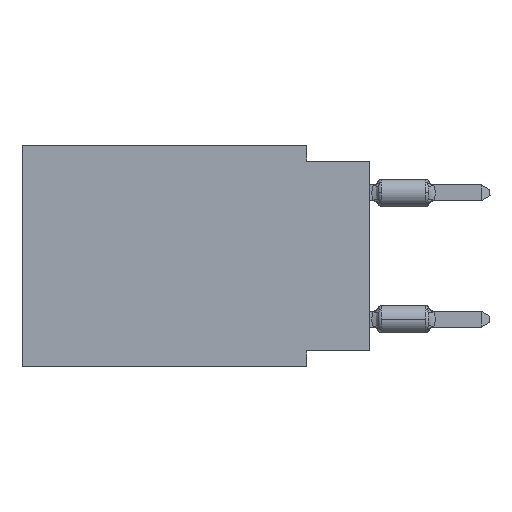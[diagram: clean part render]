
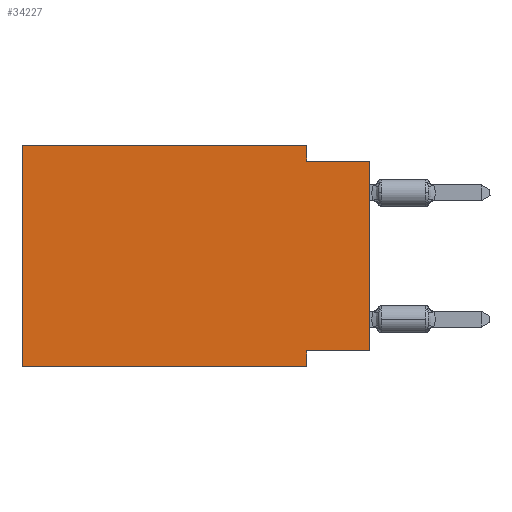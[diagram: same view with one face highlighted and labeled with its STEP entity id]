
A CAD part, left-side view. The second image highlights one B-rep face of the part: STEP entity #34227.
In plain terms, the highlighted planar face has unit normal (-1, 0, 0).
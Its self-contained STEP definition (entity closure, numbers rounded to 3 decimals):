
#984 = EDGE_CURVE ( 'NONE', #47885, #24901, #5481, .T. ) ;
#1467 = LINE ( 'NONE', #22035, #21610 ) ;
#1896 = PLANE ( 'NONE',  #51335 ) ;
#1960 = VERTEX_POINT ( 'NONE', #10460 ) ;
#2420 = FACE_OUTER_BOUND ( 'NONE', #35172, .T. ) ;
#2881 = VECTOR ( 'NONE', #37565, 1000. ) ;
#5127 = CARTESIAN_POINT ( 'NONE',  ( 0., 0., 0. ) ) ;
#5481 = LINE ( 'NONE', #21591, #23603 ) ;
#6305 = EDGE_CURVE ( 'NONE', #47885, #1960, #35040, .T. ) ;
#7955 = CARTESIAN_POINT ( 'NONE',  ( 0., 0., -0.635 ) ) ;
#8217 = CARTESIAN_POINT ( 'NONE',  ( 0., 0., -0.635 ) ) ;
#8836 = CARTESIAN_POINT ( 'NONE',  ( 0., 13.97, 0. ) ) ;
#9894 = DIRECTION ( 'NONE',  ( 0., 0., -1. ) ) ;
#10460 = CARTESIAN_POINT ( 'NONE',  ( 0., 2.54, -8.89 ) ) ;
#12663 = DIRECTION ( 'NONE',  ( 0., -1., 0. ) ) ;
#13240 = VERTEX_POINT ( 'NONE', #26535 ) ;
#14317 = EDGE_CURVE ( 'NONE', #24901, #13240, #45087, .T. ) ;
#15004 = DIRECTION ( 'NONE',  ( 0., -1., 0. ) ) ;
#16080 = CARTESIAN_POINT ( 'NONE',  ( 0., 0., -8.255 ) ) ;
#16632 = LINE ( 'NONE', #7955, #48395 ) ;
#17986 = DIRECTION ( 'NONE',  ( 1., 0., 0. ) ) ;
#18760 = DIRECTION ( 'NONE',  ( 0., 0., -1. ) ) ;
#19625 = ORIENTED_EDGE ( 'NONE', *, *, #52120, .F. ) ;
#21578 = ORIENTED_EDGE ( 'NONE', *, *, #48384, .T. ) ;
#21591 = CARTESIAN_POINT ( 'NONE',  ( 0., 13.97, 0. ) ) ;
#21610 = VECTOR ( 'NONE', #9894, 1000. ) ;
#22035 = CARTESIAN_POINT ( 'NONE',  ( 0., 2.54, -8.89 ) ) ;
#22953 = VERTEX_POINT ( 'NONE', #30923 ) ;
#23477 = VERTEX_POINT ( 'NONE', #35469 ) ;
#23603 = VECTOR ( 'NONE', #37654, 1000. ) ;
#24901 = VERTEX_POINT ( 'NONE', #8836 ) ;
#26535 = CARTESIAN_POINT ( 'NONE',  ( 0., 2.54, 0. ) ) ;
#26608 = ORIENTED_EDGE ( 'NONE', *, *, #14317, .F. ) ;
#27231 = VECTOR ( 'NONE', #39795, 1000. ) ;
#28742 = CARTESIAN_POINT ( 'NONE',  ( 0., 13.97, 0. ) ) ;
#28998 = CARTESIAN_POINT ( 'NONE',  ( 0., 2.54, 0. ) ) ;
#29066 = ORIENTED_EDGE ( 'NONE', *, *, #6305, .T. ) ;
#30370 = CARTESIAN_POINT ( 'NONE',  ( 0., 13.97, 0. ) ) ;
#30923 = CARTESIAN_POINT ( 'NONE',  ( 0., 0., -8.255 ) ) ;
#30960 = EDGE_CURVE ( 'NONE', #13240, #40230, #44571, .T. ) ;
#32254 = VECTOR ( 'NONE', #44322, 1000. ) ;
#34227 = ADVANCED_FACE ( 'NONE', ( #2420 ), #1896, .F. ) ;
#35040 = LINE ( 'NONE', #51127, #40629 ) ;
#35172 = EDGE_LOOP ( 'NONE', ( #21578, #46836, #45667, #26608, #40402, #29066, #50045, #19625 ) ) ;
#35174 = VECTOR ( 'NONE', #44828, 1000. ) ;
#35469 = CARTESIAN_POINT ( 'NONE',  ( 0., 2.54, -8.255 ) ) ;
#36360 = LINE ( 'NONE', #16080, #27231 ) ;
#37565 = DIRECTION ( 'NONE',  ( 0., 0., 1. ) ) ;
#37654 = DIRECTION ( 'NONE',  ( 0., 0., 1. ) ) ;
#39795 = DIRECTION ( 'NONE',  ( 0., 1., 0. ) ) ;
#40230 = VERTEX_POINT ( 'NONE', #41016 ) ;
#40402 = ORIENTED_EDGE ( 'NONE', *, *, #984, .F. ) ;
#40423 = EDGE_CURVE ( 'NONE', #23477, #1960, #1467, .T. ) ;
#40629 = VECTOR ( 'NONE', #15004, 1000. ) ;
#41016 = CARTESIAN_POINT ( 'NONE',  ( 0., 2.54, -0.635 ) ) ;
#44267 = CARTESIAN_POINT ( 'NONE',  ( 0., 13.97, -8.89 ) ) ;
#44322 = DIRECTION ( 'NONE',  ( 0., 0., -1. ) ) ;
#44571 = LINE ( 'NONE', #28998, #32254 ) ;
#44828 = DIRECTION ( 'NONE',  ( 0., -1., 0. ) ) ;
#45087 = LINE ( 'NONE', #28742, #35174 ) ;
#45667 = ORIENTED_EDGE ( 'NONE', *, *, #30960, .F. ) ;
#46836 = ORIENTED_EDGE ( 'NONE', *, *, #49039, .F. ) ;
#47885 = VERTEX_POINT ( 'NONE', #44267 ) ;
#48384 = EDGE_CURVE ( 'NONE', #22953, #49115, #49432, .T. ) ;
#48395 = VECTOR ( 'NONE', #12663, 1000. ) ;
#49039 = EDGE_CURVE ( 'NONE', #40230, #49115, #16632, .T. ) ;
#49115 = VERTEX_POINT ( 'NONE', #8217 ) ;
#49432 = LINE ( 'NONE', #5127, #2881 ) ;
#50045 = ORIENTED_EDGE ( 'NONE', *, *, #40423, .F. ) ;
#51127 = CARTESIAN_POINT ( 'NONE',  ( 0., 13.97, -8.89 ) ) ;
#51335 = AXIS2_PLACEMENT_3D ( 'NONE', #30370, #17986, #18760 ) ;
#52120 = EDGE_CURVE ( 'NONE', #22953, #23477, #36360, .T. ) ;
